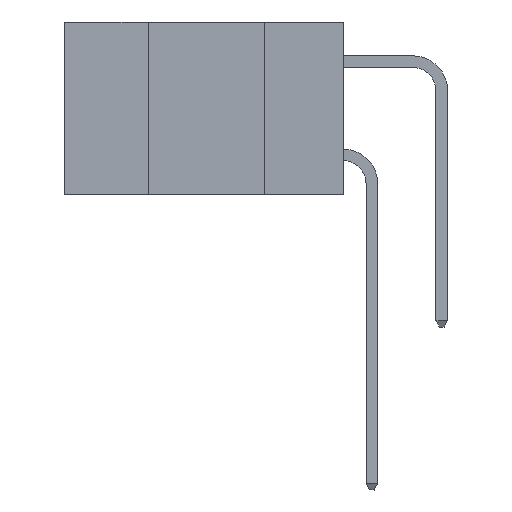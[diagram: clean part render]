
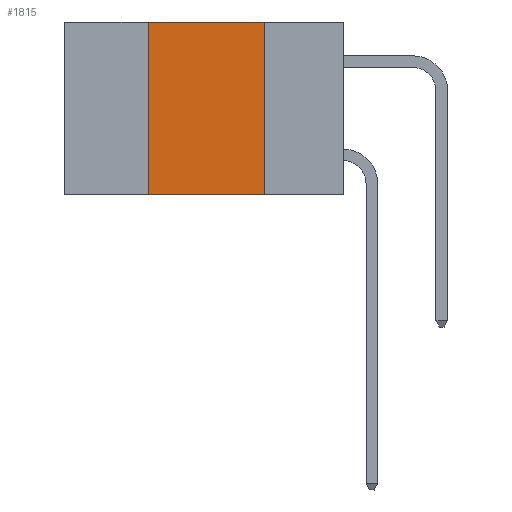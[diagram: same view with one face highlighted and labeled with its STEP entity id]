
A CAD part, left-side view. The second image highlights one B-rep face of the part: STEP entity #1815.
In plain terms, the highlighted planar face has unit normal (-1, 0, 0).
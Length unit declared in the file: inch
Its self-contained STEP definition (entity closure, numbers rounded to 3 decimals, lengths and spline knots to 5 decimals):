
#1291 = CARTESIAN_POINT ( 'NONE',  ( 0., 0.17, -0.37 ) ) ;
#1757 = EDGE_LOOP ( 'NONE', ( #9235, #19376, #21922, #20094 ) ) ;
#1815 = ADVANCED_FACE ( 'NONE', ( #20848 ), #27587, .F. ) ;
#3646 = DIRECTION ( 'NONE',  ( 0., 0., -1. ) ) ;
#4480 = VECTOR ( 'NONE', #26730, 39.37008 ) ;
#6791 = LINE ( 'NONE', #22190, #4480 ) ;
#7113 = DIRECTION ( 'NONE',  ( 0., 0., 1. ) ) ;
#7316 = CARTESIAN_POINT ( 'NONE',  ( 0., 0.17, -0.37 ) ) ;
#8345 = VECTOR ( 'NONE', #27254, 39.37008 ) ;
#9235 = ORIENTED_EDGE ( 'NONE', *, *, #10283, .F. ) ;
#9388 = CARTESIAN_POINT ( 'NONE',  ( 0., 0.6, 0. ) ) ;
#10014 = DIRECTION ( 'NONE',  ( 1., 0., 0. ) ) ;
#10283 = EDGE_CURVE ( 'NONE', #25020, #27648, #21276, .T. ) ;
#13139 = EDGE_CURVE ( 'NONE', #25508, #25020, #21233, .T. ) ;
#13867 = CARTESIAN_POINT ( 'NONE',  ( 0., 0.42, 0. ) ) ;
#14076 = VERTEX_POINT ( 'NONE', #21176 ) ;
#14793 = VECTOR ( 'NONE', #7113, 39.37008 ) ;
#15111 = CARTESIAN_POINT ( 'NONE',  ( 0., 0.17, 0. ) ) ;
#18266 = LINE ( 'NONE', #22503, #14793 ) ;
#19056 = VECTOR ( 'NONE', #3646, 39.37008 ) ;
#19376 = ORIENTED_EDGE ( 'NONE', *, *, #13139, .F. ) ;
#20094 = ORIENTED_EDGE ( 'NONE', *, *, #25499, .T. ) ;
#20848 = FACE_OUTER_BOUND ( 'NONE', #1757, .T. ) ;
#20997 = CARTESIAN_POINT ( 'NONE',  ( 0., 0.6, 0. ) ) ;
#21176 = CARTESIAN_POINT ( 'NONE',  ( 0., 0.42, -0.37 ) ) ;
#21233 = LINE ( 'NONE', #9388, #8345 ) ;
#21276 = LINE ( 'NONE', #1291, #19056 ) ;
#21922 = ORIENTED_EDGE ( 'NONE', *, *, #22676, .F. ) ;
#22190 = CARTESIAN_POINT ( 'NONE',  ( 0., 0.6, -0.37 ) ) ;
#22503 = CARTESIAN_POINT ( 'NONE',  ( 0., 0.42, -0.37 ) ) ;
#22676 = EDGE_CURVE ( 'NONE', #14076, #25508, #18266, .T. ) ;
#25020 = VERTEX_POINT ( 'NONE', #15111 ) ;
#25388 = DIRECTION ( 'NONE',  ( 0., 0., -1. ) ) ;
#25499 = EDGE_CURVE ( 'NONE', #14076, #27648, #6791, .T. ) ;
#25508 = VERTEX_POINT ( 'NONE', #13867 ) ;
#25560 = AXIS2_PLACEMENT_3D ( 'NONE', #20997, #10014, #25388 ) ;
#26730 = DIRECTION ( 'NONE',  ( 0., -1., 0. ) ) ;
#27254 = DIRECTION ( 'NONE',  ( 0., -1., 0. ) ) ;
#27587 = PLANE ( 'NONE',  #25560 ) ;
#27648 = VERTEX_POINT ( 'NONE', #7316 ) ;
